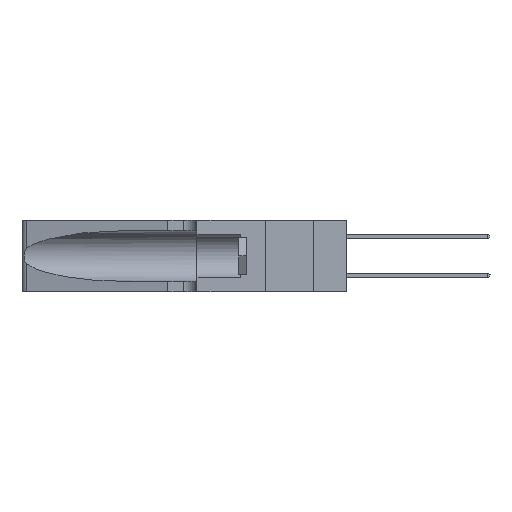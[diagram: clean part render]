
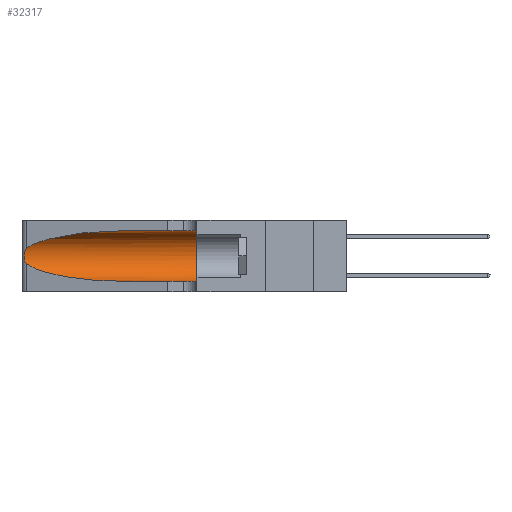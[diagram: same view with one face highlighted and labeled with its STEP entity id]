
A CAD part, left-side view. The second image highlights one B-rep face of the part: STEP entity #32317.
In plain terms, the highlighted cylindrical face has radius 3.308 mm (diameter 6.617 mm), a partial arc.
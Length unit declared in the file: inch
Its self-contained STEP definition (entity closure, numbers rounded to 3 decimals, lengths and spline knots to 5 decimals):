
#609 = EDGE_CURVE ( 'NONE', #10059, #36493, #39197, .T. ) ;
#677 = EDGE_CURVE ( 'NONE', #45005, #20156, #31058, .T. ) ;
#683 = DIRECTION ( 'NONE',  ( 0., -1., 0. ) ) ;
#1022 = CARTESIAN_POINT ( 'NONE',  ( 0.2373, 1.15595, 0.28018 ) ) ;
#1484 = EDGE_LOOP ( 'NONE', ( #9835, #37401, #12660, #7094, #36324, #36878 ) ) ;
#2588 = VECTOR ( 'NONE', #4974, 39.37008 ) ;
#2994 = CARTESIAN_POINT ( 'NONE',  ( 0.25856, 1.23593, 0.16098 ) ) ;
#4974 = DIRECTION ( 'NONE',  ( 0., -1., 0. ) ) ;
#5663 = CARTESIAN_POINT ( 'NONE',  ( 0.1305, 0.72297, 0.05475 ) ) ;
#5824 = AXIS2_PLACEMENT_3D ( 'NONE', #21946, #683, #42952 ) ;
#6576 = CARTESIAN_POINT ( 'NONE',  ( 0.25639, 1.23186, 0.15144 ) ) ;
#6688 = CIRCLE ( 'NONE', #10497, 0.13025 ) ;
#7094 = ORIENTED_EDGE ( 'NONE', *, *, #7288, .T. ) ;
#7177 = CARTESIAN_POINT ( 'NONE',  ( 0.18966, 0.96281, 0.31525 ) ) ;
#7288 = EDGE_CURVE ( 'NONE', #36493, #39144, #22602, .T. ) ;
#8290 = VERTEX_POINT ( 'NONE', #44936 ) ;
#9164 = CARTESIAN_POINT ( 'NONE',  ( 0.25487, 1.22718, 0.14631 ) ) ;
#9835 = ORIENTED_EDGE ( 'NONE', *, *, #677, .T. ) ;
#10059 = VERTEX_POINT ( 'NONE', #9164 ) ;
#10178 = CARTESIAN_POINT ( 'NONE',  ( 0.25487, 1.22718, 0.14631 ) ) ;
#10324 = EDGE_CURVE ( 'NONE', #20156, #10059, #43942, .T. ) ;
#10497 = AXIS2_PLACEMENT_3D ( 'NONE', #16651, #41216, #20192 ) ;
#11603 = CARTESIAN_POINT ( 'NONE',  ( 0.1305, 0.72297, 0.31525 ) ) ;
#12660 = ORIENTED_EDGE ( 'NONE', *, *, #609, .T. ) ;
#13613 = CARTESIAN_POINT ( 'NONE',  ( 0.25639, 1.23184, 0.21858 ) ) ;
#13701 = CARTESIAN_POINT ( 'NONE',  ( 0.25487, 1.22718, 0.22369 ) ) ;
#14347 = CARTESIAN_POINT ( 'NONE',  ( 0.25487, 1.22718, 0.22369 ) ) ;
#16651 = CARTESIAN_POINT ( 'NONE',  ( 0.1305, 0.35, 0.185 ) ) ;
#17151 = CARTESIAN_POINT ( 'NONE',  ( 0.25854, 1.2359, 0.20912 ) ) ;
#17418 = CARTESIAN_POINT ( 'NONE',  ( 0.25487, 1.22718, 0.14631 ) ) ;
#20156 = VERTEX_POINT ( 'NONE', #13701 ) ;
#20192 = DIRECTION ( 'NONE',  ( 0., 0., 1. ) ) ;
#20605 = CARTESIAN_POINT ( 'NONE',  ( 0.1305, 1.61858, 0.31525 ) ) ;
#20682 = CARTESIAN_POINT ( 'NONE',  ( 0.26075, 1.23896, 0.19203 ) ) ;
#21946 = CARTESIAN_POINT ( 'NONE',  ( 0.1305, 1.61858, 0.185 ) ) ;
#22602 = LINE ( 'NONE', #22671, #2588 ) ;
#22671 = CARTESIAN_POINT ( 'NONE',  ( 0.1305, 1.61858, 0.05475 ) ) ;
#24078 = CARTESIAN_POINT ( 'NONE',  ( 0.25487, 1.22718, 0.22369 ) ) ;
#24232 = CARTESIAN_POINT ( 'NONE',  ( 0.26017, 1.23833, 0.17102 ) ) ;
#26101 = FACE_OUTER_BOUND ( 'NONE', #1484, .T. ) ;
#27375 = VECTOR ( 'NONE', #41641, 39.37008 ) ;
#27616 = CARTESIAN_POINT ( 'NONE',  ( 0.25555, 1.22994, 0.2215 ) ) ;
#27770 = CARTESIAN_POINT ( 'NONE',  ( 0.25789, 1.23486, 0.15765 ) ) ;
#31058 =( BOUNDED_CURVE ( )  B_SPLINE_CURVE ( 3, ( #35422, #7177, #1022, #14347 ),
 .UNSPECIFIED., .F., .T. ) 
 B_SPLINE_CURVE_WITH_KNOTS ( ( 4, 4 ),
 ( 1.5708, 2.84003 ),
 .UNSPECIFIED. ) 
 CURVE ( )  GEOMETRIC_REPRESENTATION_ITEM ( )  RATIONAL_B_SPLINE_CURVE ( ( 1., 0.87, 0.87, 1. ) ) 
 REPRESENTATION_ITEM ( '' )  );
#31330 = CARTESIAN_POINT ( 'NONE',  ( 0.25555, 1.22993, 0.14849 ) ) ;
#31434 = CARTESIAN_POINT ( 'NONE',  ( 0.1305, 0.35, 0.05475 ) ) ;
#32317 = ADVANCED_FACE ( 'NONE', ( #26101 ), #43648, .F. ) ;
#34954 = CARTESIAN_POINT ( 'NONE',  ( 0.2373, 1.15595, 0.08982 ) ) ;
#35422 = CARTESIAN_POINT ( 'NONE',  ( 0.1305, 0.72297, 0.31525 ) ) ;
#36324 = ORIENTED_EDGE ( 'NONE', *, *, #38978, .F. ) ;
#36493 = VERTEX_POINT ( 'NONE', #5663 ) ;
#36878 = ORIENTED_EDGE ( 'NONE', *, *, #42386, .F. ) ;
#37401 = ORIENTED_EDGE ( 'NONE', *, *, #10324, .T. ) ;
#37817 = LINE ( 'NONE', #20605, #27375 ) ;
#38182 = CARTESIAN_POINT ( 'NONE',  ( 0.25787, 1.23484, 0.2124 ) ) ;
#38978 = EDGE_CURVE ( 'NONE', #8290, #39144, #6688, .T. ) ;
#39144 = VERTEX_POINT ( 'NONE', #31434 ) ;
#39197 =( BOUNDED_CURVE ( )  B_SPLINE_CURVE ( 3, ( #17418, #34954, #41828, #41972 ),
 .UNSPECIFIED., .F., .F. ) 
 B_SPLINE_CURVE_WITH_KNOTS ( ( 4, 4 ),
 ( 3.44316, 4.71239 ),
 .UNSPECIFIED. ) 
 CURVE ( )  GEOMETRIC_REPRESENTATION_ITEM ( )  RATIONAL_B_SPLINE_CURVE ( ( 1., 0.87, 0.87, 1. ) ) 
 REPRESENTATION_ITEM ( '' )  );
#41216 = DIRECTION ( 'NONE',  ( 0., 1., 0. ) ) ;
#41641 = DIRECTION ( 'NONE',  ( 0., -1., 0. ) ) ;
#41708 = CARTESIAN_POINT ( 'NONE',  ( 0.26018, 1.23835, 0.19895 ) ) ;
#41828 = CARTESIAN_POINT ( 'NONE',  ( 0.18966, 0.96281, 0.05475 ) ) ;
#41972 = CARTESIAN_POINT ( 'NONE',  ( 0.1305, 0.72297, 0.05475 ) ) ;
#42386 = EDGE_CURVE ( 'NONE', #45005, #8290, #37817, .T. ) ;
#42952 = DIRECTION ( 'NONE',  ( 0., 0., -1. ) ) ;
#43648 = CYLINDRICAL_SURFACE ( 'NONE', #5824, 0.13025 ) ;
#43942 = B_SPLINE_CURVE_WITH_KNOTS ( 'NONE', 3,
 ( #24078, #27616, #13613, #38182, #17151, #41708, #20682, #45214, #24232, #2994, #27770, #6576, #31330, #10178 ),
 .UNSPECIFIED., .F., .F.,
 ( 4, 2, 2, 2, 2, 2, 4 ),
 ( 0., 0.00027, 0.00053, 0.00107, 0.0016, 0.00187, 0.00214 ),
 .UNSPECIFIED. ) ;
#44936 = CARTESIAN_POINT ( 'NONE',  ( 0.1305, 0.35, 0.31525 ) ) ;
#45005 = VERTEX_POINT ( 'NONE', #11603 ) ;
#45214 = CARTESIAN_POINT ( 'NONE',  ( 0.26075, 1.23896, 0.178 ) ) ;
